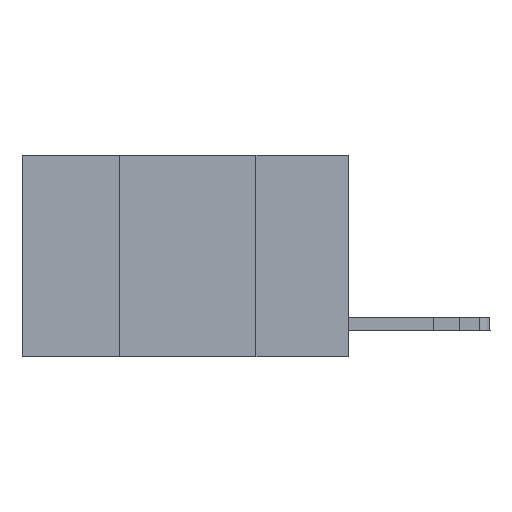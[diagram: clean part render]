
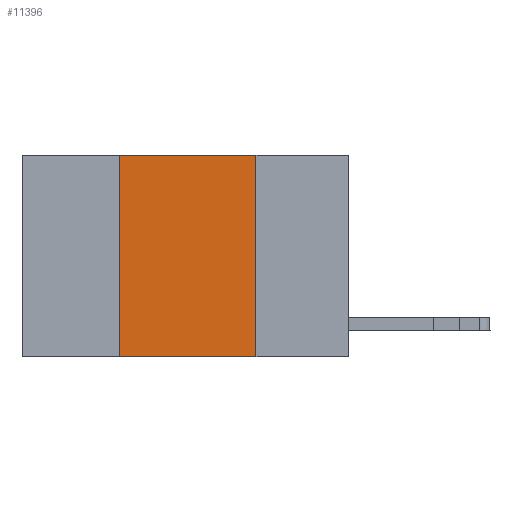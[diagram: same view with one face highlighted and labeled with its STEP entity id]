
A CAD part, left-side view. The second image highlights one B-rep face of the part: STEP entity #11396.
In plain terms, the highlighted planar face has unit normal (-1, 0, 0).
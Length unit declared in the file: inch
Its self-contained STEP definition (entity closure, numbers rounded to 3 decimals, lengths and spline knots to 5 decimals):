
#554 = LINE ( 'NONE', #3313, #4042 ) ;
#698 = DIRECTION ( 'NONE',  ( 0., 0., -1. ) ) ;
#1349 = ORIENTED_EDGE ( 'NONE', *, *, #5905, .F. ) ;
#2273 = EDGE_CURVE ( 'NONE', #7698, #9202, #7817, .T. ) ;
#2292 = VECTOR ( 'NONE', #5559, 39.37008 ) ;
#2542 = VECTOR ( 'NONE', #9561, 39.37008 ) ;
#2586 = CARTESIAN_POINT ( 'NONE',  ( 0., 0.42, -0.37 ) ) ;
#2677 = LINE ( 'NONE', #9844, #2542 ) ;
#2883 = LINE ( 'NONE', #13966, #2292 ) ;
#3313 = CARTESIAN_POINT ( 'NONE',  ( 0., 0.6, -0.37 ) ) ;
#3397 = DIRECTION ( 'NONE',  ( 0., -1., 0. ) ) ;
#3447 = CARTESIAN_POINT ( 'NONE',  ( 0., 0.6, 0. ) ) ;
#3509 = CARTESIAN_POINT ( 'NONE',  ( 0., 0.6, 0. ) ) ;
#4042 = VECTOR ( 'NONE', #3397, 39.37008 ) ;
#5559 = DIRECTION ( 'NONE',  ( 0., 0., 1. ) ) ;
#5905 = EDGE_CURVE ( 'NONE', #9202, #15463, #2677, .T. ) ;
#6538 = ORIENTED_EDGE ( 'NONE', *, *, #2273, .F. ) ;
#6615 = EDGE_CURVE ( 'NONE', #17329, #15463, #554, .T. ) ;
#6825 = ORIENTED_EDGE ( 'NONE', *, *, #6615, .T. ) ;
#7698 = VERTEX_POINT ( 'NONE', #10899 ) ;
#7817 = LINE ( 'NONE', #3509, #9481 ) ;
#8002 = DIRECTION ( 'NONE',  ( 0., -1., 0. ) ) ;
#9038 = DIRECTION ( 'NONE',  ( 1., 0., 0. ) ) ;
#9202 = VERTEX_POINT ( 'NONE', #11195 ) ;
#9481 = VECTOR ( 'NONE', #8002, 39.37008 ) ;
#9561 = DIRECTION ( 'NONE',  ( 0., 0., -1. ) ) ;
#9844 = CARTESIAN_POINT ( 'NONE',  ( 0., 0.17, 0. ) ) ;
#10403 = FACE_OUTER_BOUND ( 'NONE', #14700, .T. ) ;
#10713 = AXIS2_PLACEMENT_3D ( 'NONE', #3447, #9038, #698 ) ;
#10899 = CARTESIAN_POINT ( 'NONE',  ( 0., 0.42, 0. ) ) ;
#11195 = CARTESIAN_POINT ( 'NONE',  ( 0., 0.17, 0. ) ) ;
#11396 = ADVANCED_FACE ( 'NONE', ( #10403 ), #15987, .F. ) ;
#13966 = CARTESIAN_POINT ( 'NONE',  ( 0., 0.42, 0. ) ) ;
#13971 = EDGE_CURVE ( 'NONE', #17329, #7698, #2883, .T. ) ;
#14621 = CARTESIAN_POINT ( 'NONE',  ( 0., 0.17, -0.37 ) ) ;
#14700 = EDGE_LOOP ( 'NONE', ( #1349, #6538, #16952, #6825 ) ) ;
#15463 = VERTEX_POINT ( 'NONE', #14621 ) ;
#15987 = PLANE ( 'NONE',  #10713 ) ;
#16952 = ORIENTED_EDGE ( 'NONE', *, *, #13971, .F. ) ;
#17329 = VERTEX_POINT ( 'NONE', #2586 ) ;
